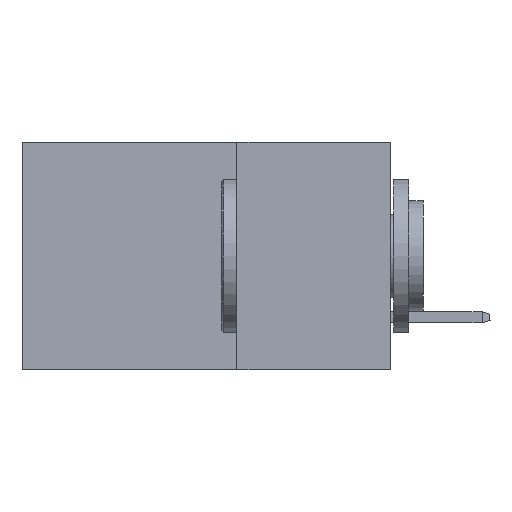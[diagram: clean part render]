
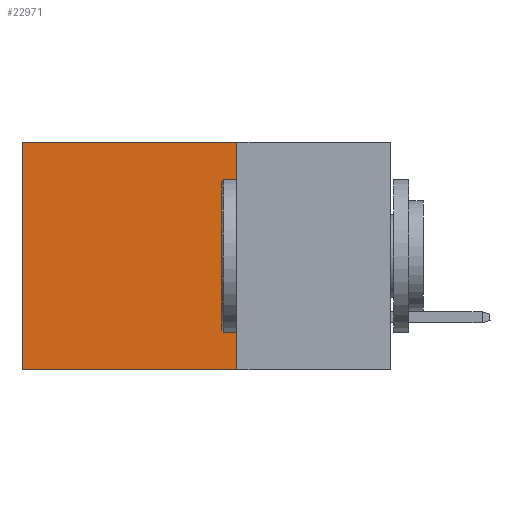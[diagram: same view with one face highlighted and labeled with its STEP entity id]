
A CAD part, left-side view. The second image highlights one B-rep face of the part: STEP entity #22971.
In plain terms, the highlighted planar face has unit normal (-1, 0, 0).
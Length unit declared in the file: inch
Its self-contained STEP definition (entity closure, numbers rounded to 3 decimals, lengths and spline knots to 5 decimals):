
#225 = VERTEX_POINT ( 'NONE', #27824 ) ;
#1043 = EDGE_LOOP ( 'NONE', ( #14019, #26831, #10033, #9071 ) ) ;
#1143 = DIRECTION ( 'NONE',  ( 0., 0., -1. ) ) ;
#1554 = EDGE_CURVE ( 'NONE', #9843, #23244, #18011, .T. ) ;
#2105 = FACE_OUTER_BOUND ( 'NONE', #1043, .T. ) ;
#3315 = AXIS2_PLACEMENT_3D ( 'NONE', #8681, #10662, #15798 ) ;
#6201 = CARTESIAN_POINT ( 'NONE',  ( 0.2875, 0.25, -0.37 ) ) ;
#7625 = VECTOR ( 'NONE', #13704, 39.37008 ) ;
#8082 = EDGE_CURVE ( 'NONE', #225, #9843, #17902, .T. ) ;
#8130 = VECTOR ( 'NONE', #1143, 39.37008 ) ;
#8681 = CARTESIAN_POINT ( 'NONE',  ( 0.2875, 0.25, 0. ) ) ;
#9071 = ORIENTED_EDGE ( 'NONE', *, *, #8082, .T. ) ;
#9214 = CARTESIAN_POINT ( 'NONE',  ( 0.2875, 0.6, 0. ) ) ;
#9843 = VERTEX_POINT ( 'NONE', #9214 ) ;
#10033 = ORIENTED_EDGE ( 'NONE', *, *, #13668, .F. ) ;
#10462 = EDGE_CURVE ( 'NONE', #24933, #23244, #14524, .T. ) ;
#10662 = DIRECTION ( 'NONE',  ( 1., 0., 0. ) ) ;
#10882 = VECTOR ( 'NONE', #30782, 39.37008 ) ;
#13562 = CARTESIAN_POINT ( 'NONE',  ( 0.2875, 0.6, 0. ) ) ;
#13604 = CARTESIAN_POINT ( 'NONE',  ( 0.2875, 0.25, -0.37 ) ) ;
#13648 = CARTESIAN_POINT ( 'NONE',  ( 0.2875, 0.25, 0. ) ) ;
#13668 = EDGE_CURVE ( 'NONE', #225, #24933, #27000, .T. ) ;
#13704 = DIRECTION ( 'NONE',  ( 0., 1., 0. ) ) ;
#14019 = ORIENTED_EDGE ( 'NONE', *, *, #1554, .T. ) ;
#14524 = LINE ( 'NONE', #13604, #7625 ) ;
#15798 = DIRECTION ( 'NONE',  ( 0., 0., -1. ) ) ;
#17902 = LINE ( 'NONE', #19842, #25611 ) ;
#18011 = LINE ( 'NONE', #13562, #8130 ) ;
#19542 = DIRECTION ( 'NONE',  ( 0., 1., 0. ) ) ;
#19842 = CARTESIAN_POINT ( 'NONE',  ( 0.2875, 0.25, 0. ) ) ;
#22971 = ADVANCED_FACE ( 'NONE', ( #2105 ), #25447, .F. ) ;
#23244 = VERTEX_POINT ( 'NONE', #28154 ) ;
#24933 = VERTEX_POINT ( 'NONE', #6201 ) ;
#25447 = PLANE ( 'NONE',  #3315 ) ;
#25611 = VECTOR ( 'NONE', #19542, 39.37008 ) ;
#26831 = ORIENTED_EDGE ( 'NONE', *, *, #10462, .F. ) ;
#27000 = LINE ( 'NONE', #13648, #10882 ) ;
#27824 = CARTESIAN_POINT ( 'NONE',  ( 0.2875, 0.25, 0. ) ) ;
#28154 = CARTESIAN_POINT ( 'NONE',  ( 0.2875, 0.6, -0.37 ) ) ;
#30782 = DIRECTION ( 'NONE',  ( 0., 0., -1. ) ) ;
